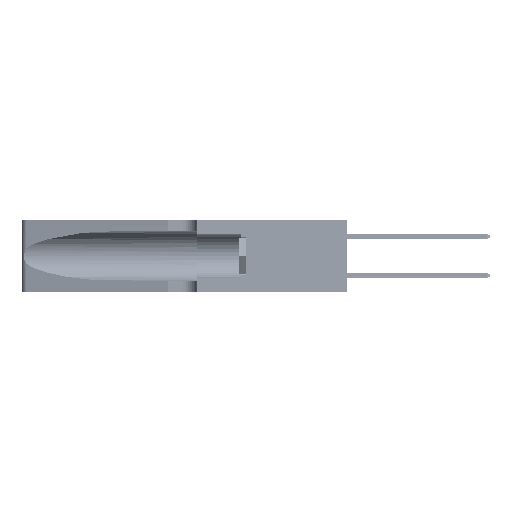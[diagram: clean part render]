
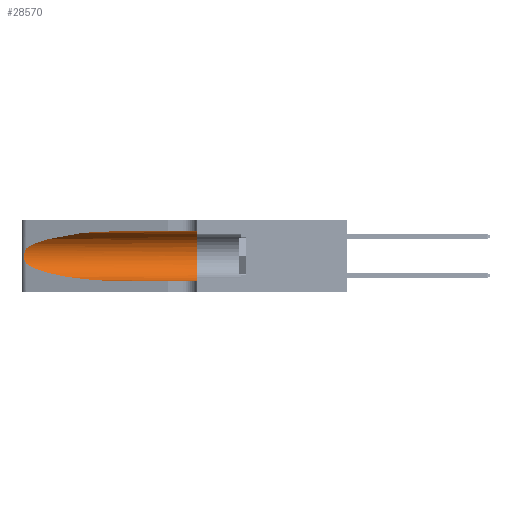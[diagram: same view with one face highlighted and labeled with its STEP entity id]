
A CAD part, left-side view. The second image highlights one B-rep face of the part: STEP entity #28570.
In plain terms, the highlighted cylindrical face has radius 3.308 mm (diameter 6.617 mm), a partial arc.
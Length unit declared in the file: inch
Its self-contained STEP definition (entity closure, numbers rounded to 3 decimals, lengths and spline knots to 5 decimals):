
#625 = CARTESIAN_POINT ( 'NONE',  ( 0.25856, 1.23593, 0.16098 ) ) ;
#730 = LINE ( 'NONE', #40362, #3118 ) ;
#791 = CARTESIAN_POINT ( 'NONE',  ( 0.25487, 1.22718, 0.22369 ) ) ;
#1244 = VERTEX_POINT ( 'NONE', #4603 ) ;
#1475 = CARTESIAN_POINT ( 'NONE',  ( 0.25487, 1.22718, 0.14631 ) ) ;
#3118 = VECTOR ( 'NONE', #13856, 39.37008 ) ;
#3946 = CARTESIAN_POINT ( 'NONE',  ( 0.25487, 1.22718, 0.14631 ) ) ;
#4458 = CARTESIAN_POINT ( 'NONE',  ( 0.25639, 1.23186, 0.15144 ) ) ;
#4603 = CARTESIAN_POINT ( 'NONE',  ( 0.25487, 1.22718, 0.14631 ) ) ;
#5329 = CARTESIAN_POINT ( 'NONE',  ( 0.18966, 0.96281, 0.05475 ) ) ;
#6836 = CARTESIAN_POINT ( 'NONE',  ( 0.18966, 0.96281, 0.31525 ) ) ;
#7110 = EDGE_CURVE ( 'NONE', #11309, #35679, #43751, .T. ) ;
#9518 = EDGE_LOOP ( 'NONE', ( #19780, #37752, #41674, #40383, #26693, #14465 ) ) ;
#10081 = CARTESIAN_POINT ( 'NONE',  ( 0.1305, 0.35, 0.31525 ) ) ;
#10209 = DIRECTION ( 'NONE',  ( 0., 1., 0. ) ) ;
#11309 = VERTEX_POINT ( 'NONE', #16580 ) ;
#11515 = CARTESIAN_POINT ( 'NONE',  ( 0.25787, 1.23484, 0.2124 ) ) ;
#11548 = EDGE_CURVE ( 'NONE', #41746, #28081, #40720, .T. ) ;
#11936 = CARTESIAN_POINT ( 'NONE',  ( 0.1305, 1.61858, 0.05475 ) ) ;
#13856 = DIRECTION ( 'NONE',  ( 0., -1., 0. ) ) ;
#14465 = ORIENTED_EDGE ( 'NONE', *, *, #44756, .F. ) ;
#14818 = VERTEX_POINT ( 'NONE', #10081 ) ;
#15340 = CARTESIAN_POINT ( 'NONE',  ( 0.26018, 1.23835, 0.19895 ) ) ;
#15506 = CARTESIAN_POINT ( 'NONE',  ( 0.25555, 1.22993, 0.14849 ) ) ;
#15680 = CARTESIAN_POINT ( 'NONE',  ( 0.26075, 1.23896, 0.178 ) ) ;
#16580 = CARTESIAN_POINT ( 'NONE',  ( 0.1305, 0.72297, 0.05475 ) ) ;
#16915 = DIRECTION ( 'NONE',  ( 0., 0., -1. ) ) ;
#18898 =( BOUNDED_CURVE ( )  B_SPLINE_CURVE ( 3, ( #1475, #47504, #5329, #32094 ),
 .UNSPECIFIED., .F., .F. ) 
 B_SPLINE_CURVE_WITH_KNOTS ( ( 4, 4 ),
 ( 3.44316, 4.71239 ),
 .UNSPECIFIED. ) 
 CURVE ( )  GEOMETRIC_REPRESENTATION_ITEM ( )  RATIONAL_B_SPLINE_CURVE ( ( 1., 0.87, 0.87, 1. ) ) 
 REPRESENTATION_ITEM ( '' )  );
#19641 = DIRECTION ( 'NONE',  ( 0., -1., 0. ) ) ;
#19780 = ORIENTED_EDGE ( 'NONE', *, *, #11548, .T. ) ;
#23530 = CARTESIAN_POINT ( 'NONE',  ( 0.26017, 1.23833, 0.17102 ) ) ;
#24288 = EDGE_CURVE ( 'NONE', #14818, #35679, #31157, .T. ) ;
#26693 = ORIENTED_EDGE ( 'NONE', *, *, #24288, .F. ) ;
#26763 = AXIS2_PLACEMENT_3D ( 'NONE', #44680, #10209, #33266 ) ;
#26934 = CYLINDRICAL_SURFACE ( 'NONE', #31168, 0.13025 ) ;
#27395 = CARTESIAN_POINT ( 'NONE',  ( 0.1305, 0.35, 0.05475 ) ) ;
#28081 = VERTEX_POINT ( 'NONE', #28181 ) ;
#28181 = CARTESIAN_POINT ( 'NONE',  ( 0.25487, 1.22718, 0.22369 ) ) ;
#28570 = ADVANCED_FACE ( 'NONE', ( #43159 ), #26934, .F. ) ;
#28748 = VECTOR ( 'NONE', #19641, 39.37008 ) ;
#31157 = CIRCLE ( 'NONE', #26763, 0.13025 ) ;
#31168 = AXIS2_PLACEMENT_3D ( 'NONE', #35828, #39546, #16915 ) ;
#32094 = CARTESIAN_POINT ( 'NONE',  ( 0.1305, 0.72297, 0.05475 ) ) ;
#33266 = DIRECTION ( 'NONE',  ( 0., 0., 1. ) ) ;
#34418 = CARTESIAN_POINT ( 'NONE',  ( 0.25555, 1.22994, 0.2215 ) ) ;
#34923 = CARTESIAN_POINT ( 'NONE',  ( 0.25639, 1.23184, 0.21858 ) ) ;
#35679 = VERTEX_POINT ( 'NONE', #27395 ) ;
#35828 = CARTESIAN_POINT ( 'NONE',  ( 0.1305, 1.61858, 0.185 ) ) ;
#36366 = EDGE_CURVE ( 'NONE', #1244, #11309, #18898, .T. ) ;
#37752 = ORIENTED_EDGE ( 'NONE', *, *, #47926, .T. ) ;
#38313 = CARTESIAN_POINT ( 'NONE',  ( 0.25789, 1.23486, 0.15765 ) ) ;
#38656 = CARTESIAN_POINT ( 'NONE',  ( 0.26075, 1.23896, 0.19203 ) ) ;
#39546 = DIRECTION ( 'NONE',  ( 0., -1., 0. ) ) ;
#40362 = CARTESIAN_POINT ( 'NONE',  ( 0.1305, 1.61858, 0.31525 ) ) ;
#40383 = ORIENTED_EDGE ( 'NONE', *, *, #7110, .T. ) ;
#40720 =( BOUNDED_CURVE ( )  B_SPLINE_CURVE ( 3, ( #48691, #6836, #45031, #49191 ),
 .UNSPECIFIED., .F., .F. ) 
 B_SPLINE_CURVE_WITH_KNOTS ( ( 4, 4 ),
 ( 1.5708, 2.84003 ),
 .UNSPECIFIED. ) 
 CURVE ( )  GEOMETRIC_REPRESENTATION_ITEM ( )  RATIONAL_B_SPLINE_CURVE ( ( 1., 0.87, 0.87, 1. ) ) 
 REPRESENTATION_ITEM ( '' )  );
#41674 = ORIENTED_EDGE ( 'NONE', *, *, #36366, .T. ) ;
#41746 = VERTEX_POINT ( 'NONE', #48854 ) ;
#43159 = FACE_OUTER_BOUND ( 'NONE', #9518, .T. ) ;
#43751 = LINE ( 'NONE', #11936, #28748 ) ;
#44680 = CARTESIAN_POINT ( 'NONE',  ( 0.1305, 0.35, 0.185 ) ) ;
#44756 = EDGE_CURVE ( 'NONE', #41746, #14818, #730, .T. ) ;
#45031 = CARTESIAN_POINT ( 'NONE',  ( 0.2373, 1.15595, 0.28018 ) ) ;
#46476 = CARTESIAN_POINT ( 'NONE',  ( 0.25854, 1.2359, 0.20912 ) ) ;
#47504 = CARTESIAN_POINT ( 'NONE',  ( 0.2373, 1.15595, 0.08982 ) ) ;
#47926 = EDGE_CURVE ( 'NONE', #28081, #1244, #48048, .T. ) ;
#48048 = B_SPLINE_CURVE_WITH_KNOTS ( 'NONE', 3,
 ( #791, #34418, #34923, #11515, #46476, #15340, #38656, #15680, #23530, #625, #38313, #4458, #15506, #3946 ),
 .UNSPECIFIED., .F., .F.,
 ( 4, 2, 2, 2, 2, 2, 4 ),
 ( 0., 0.00027, 0.00053, 0.00107, 0.0016, 0.00187, 0.00214 ),
 .UNSPECIFIED. ) ;
#48691 = CARTESIAN_POINT ( 'NONE',  ( 0.1305, 0.72297, 0.31525 ) ) ;
#48854 = CARTESIAN_POINT ( 'NONE',  ( 0.1305, 0.72297, 0.31525 ) ) ;
#49191 = CARTESIAN_POINT ( 'NONE',  ( 0.25487, 1.22718, 0.22369 ) ) ;
